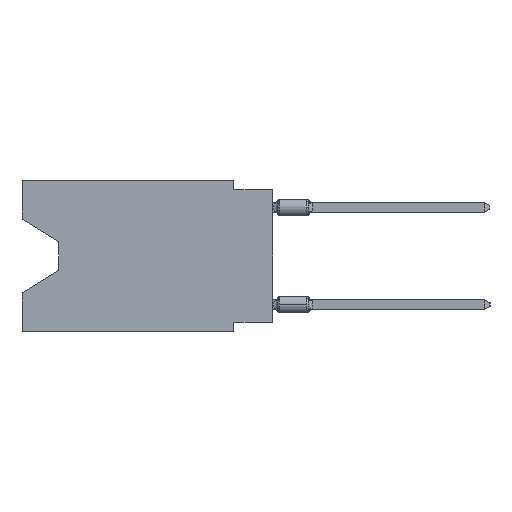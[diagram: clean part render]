
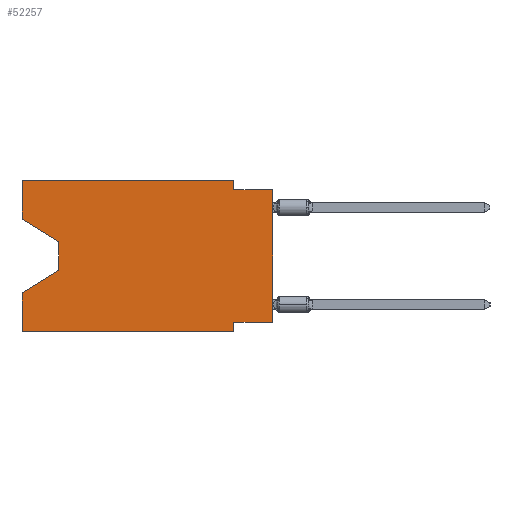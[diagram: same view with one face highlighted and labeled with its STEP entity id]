
A CAD part, left-side view. The second image highlights one B-rep face of the part: STEP entity #52257.
In plain terms, the highlighted planar face has unit normal (-1, 0, 0).
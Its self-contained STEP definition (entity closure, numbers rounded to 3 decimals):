
#366 = EDGE_CURVE ( 'NONE', #55638, #28346, #46553, .T. ) ;
#1294 = VECTOR ( 'NONE', #20960, 1000. ) ;
#1866 = VERTEX_POINT ( 'NONE', #36059 ) ;
#1870 = ORIENTED_EDGE ( 'NONE', *, *, #53201, .T. ) ;
#2819 = ORIENTED_EDGE ( 'NONE', *, *, #52890, .T. ) ;
#2922 = EDGE_CURVE ( 'NONE', #54757, #55638, #57421, .T. ) ;
#4633 = PLANE ( 'NONE',  #50530 ) ;
#4907 = DIRECTION ( 'NONE',  ( 0., -0.855, -0.519 ) ) ;
#5307 = ORIENTED_EDGE ( 'NONE', *, *, #57145, .F. ) ;
#5573 = DIRECTION ( 'NONE',  ( 0., 0., 1. ) ) ;
#8539 = EDGE_CURVE ( 'NONE', #25797, #28346, #11814, .T. ) ;
#8674 = VECTOR ( 'NONE', #58001, 1000. ) ;
#8741 = ORIENTED_EDGE ( 'NONE', *, *, #15308, .F. ) ;
#9091 = DIRECTION ( 'NONE',  ( 0., -1., 0. ) ) ;
#10360 = VECTOR ( 'NONE', #36535, 1000. ) ;
#11377 = LINE ( 'NONE', #33878, #1294 ) ;
#11814 = LINE ( 'NONE', #14172, #19852 ) ;
#13348 = LINE ( 'NONE', #13637, #20551 ) ;
#13607 = CARTESIAN_POINT ( 'NONE',  ( 0., 13.97, -5.893 ) ) ;
#13637 = CARTESIAN_POINT ( 'NONE',  ( 0., 13.97, -4.013 ) ) ;
#13999 = CARTESIAN_POINT ( 'NONE',  ( 0., 2.54, -9.271 ) ) ;
#14172 = CARTESIAN_POINT ( 'NONE',  ( 0., 16.383, -9.906 ) ) ;
#14525 = DIRECTION ( 'NONE',  ( 0., 0., -1. ) ) ;
#15308 = EDGE_CURVE ( 'NONE', #23628, #32396, #30464, .T. ) ;
#16173 = EDGE_CURVE ( 'NONE', #55126, #47197, #18011, .T. ) ;
#16391 = CARTESIAN_POINT ( 'NONE',  ( 0., 0., -9.271 ) ) ;
#16395 = CARTESIAN_POINT ( 'NONE',  ( 0., 2.54, -9.906 ) ) ;
#16447 = EDGE_CURVE ( 'NONE', #45241, #1866, #11377, .T. ) ;
#18011 = LINE ( 'NONE', #49432, #23312 ) ;
#18256 = CARTESIAN_POINT ( 'NONE',  ( 0., 2.54, -9.906 ) ) ;
#19359 = EDGE_CURVE ( 'NONE', #47197, #27373, #24805, .T. ) ;
#19852 = VECTOR ( 'NONE', #9091, 1000. ) ;
#20551 = VECTOR ( 'NONE', #14525, 1000. ) ;
#20960 = DIRECTION ( 'NONE',  ( 0., 0.855, -0.519 ) ) ;
#21456 = ORIENTED_EDGE ( 'NONE', *, *, #45015, .F. ) ;
#22072 = ORIENTED_EDGE ( 'NONE', *, *, #16447, .T. ) ;
#23112 = ORIENTED_EDGE ( 'NONE', *, *, #19359, .F. ) ;
#23312 = VECTOR ( 'NONE', #57852, 1000. ) ;
#23628 = VERTEX_POINT ( 'NONE', #31144 ) ;
#24805 = LINE ( 'NONE', #33212, #38998 ) ;
#25764 = VECTOR ( 'NONE', #4907, 1000. ) ;
#25797 = VERTEX_POINT ( 'NONE', #49208 ) ;
#27012 = VERTEX_POINT ( 'NONE', #33206 ) ;
#27245 = VECTOR ( 'NONE', #5573, 1000. ) ;
#27270 = CARTESIAN_POINT ( 'NONE',  ( 0., 16.383, -2.546 ) ) ;
#27373 = VERTEX_POINT ( 'NONE', #54974 ) ;
#28013 = VECTOR ( 'NONE', #39157, 1000. ) ;
#28346 = VERTEX_POINT ( 'NONE', #16395 ) ;
#28351 = CARTESIAN_POINT ( 'NONE',  ( 0., 16.383, 0. ) ) ;
#29977 = ORIENTED_EDGE ( 'NONE', *, *, #35208, .T. ) ;
#30464 = LINE ( 'NONE', #39748, #28013 ) ;
#31144 = CARTESIAN_POINT ( 'NONE',  ( 0., 2.54, -0.635 ) ) ;
#31283 = ORIENTED_EDGE ( 'NONE', *, *, #2922, .F. ) ;
#31454 = ORIENTED_EDGE ( 'NONE', *, *, #16173, .F. ) ;
#31615 = LINE ( 'NONE', #41485, #25764 ) ;
#32214 = DIRECTION ( 'NONE',  ( 1., 0., 0. ) ) ;
#32396 = VERTEX_POINT ( 'NONE', #38768 ) ;
#33206 = CARTESIAN_POINT ( 'NONE',  ( 0., 13.97, -4.013 ) ) ;
#33212 = CARTESIAN_POINT ( 'NONE',  ( 0., 16.383, 0. ) ) ;
#33878 = CARTESIAN_POINT ( 'NONE',  ( 0., 13.97, -5.893 ) ) ;
#34643 = CARTESIAN_POINT ( 'NONE',  ( 0., 2.54, 0. ) ) ;
#35162 = CARTESIAN_POINT ( 'NONE',  ( 0., 0., 0. ) ) ;
#35208 = EDGE_CURVE ( 'NONE', #27012, #45241, #13348, .T. ) ;
#36059 = CARTESIAN_POINT ( 'NONE',  ( 0., 16.383, -7.36 ) ) ;
#36255 = ORIENTED_EDGE ( 'NONE', *, *, #366, .F. ) ;
#36535 = DIRECTION ( 'NONE',  ( 0., 0., -1. ) ) ;
#38768 = CARTESIAN_POINT ( 'NONE',  ( 0., 0., -0.635 ) ) ;
#38841 = DIRECTION ( 'NONE',  ( 0., 0., -1. ) ) ;
#38998 = VECTOR ( 'NONE', #43061, 1000. ) ;
#39157 = DIRECTION ( 'NONE',  ( 0., -1., 0. ) ) ;
#39356 = DIRECTION ( 'NONE',  ( 0., 0., 1. ) ) ;
#39748 = CARTESIAN_POINT ( 'NONE',  ( 0., 0., -0.635 ) ) ;
#41485 = CARTESIAN_POINT ( 'NONE',  ( 0., 16.383, -2.546 ) ) ;
#42362 = VECTOR ( 'NONE', #38841, 1000. ) ;
#42382 = CARTESIAN_POINT ( 'NONE',  ( 0., 16.383, 0. ) ) ;
#43061 = DIRECTION ( 'NONE',  ( 0., -1., 0. ) ) ;
#43305 = LINE ( 'NONE', #28351, #27245 ) ;
#44353 = CARTESIAN_POINT ( 'NONE',  ( 0., 16.383, 0. ) ) ;
#45015 = EDGE_CURVE ( 'NONE', #25797, #1866, #43305, .T. ) ;
#45241 = VERTEX_POINT ( 'NONE', #13607 ) ;
#45657 = CARTESIAN_POINT ( 'NONE',  ( 0., 0., -9.271 ) ) ;
#45664 = FACE_OUTER_BOUND ( 'NONE', #56021, .T. ) ;
#46553 = LINE ( 'NONE', #18256, #10360 ) ;
#47197 = VERTEX_POINT ( 'NONE', #44353 ) ;
#49208 = CARTESIAN_POINT ( 'NONE',  ( 0., 16.383, -9.906 ) ) ;
#49432 = CARTESIAN_POINT ( 'NONE',  ( 0., 16.383, 0. ) ) ;
#50451 = DIRECTION ( 'NONE',  ( 0., 0., -1. ) ) ;
#50530 = AXIS2_PLACEMENT_3D ( 'NONE', #42382, #32214, #50451 ) ;
#52257 = ADVANCED_FACE ( 'NONE', ( #45664 ), #4633, .F. ) ;
#52329 = ORIENTED_EDGE ( 'NONE', *, *, #8539, .T. ) ;
#52890 = EDGE_CURVE ( 'NONE', #55126, #27012, #31615, .T. ) ;
#53201 = EDGE_CURVE ( 'NONE', #54757, #32396, #57893, .T. ) ;
#53494 = VECTOR ( 'NONE', #39356, 1000. ) ;
#54757 = VERTEX_POINT ( 'NONE', #45657 ) ;
#54974 = CARTESIAN_POINT ( 'NONE',  ( 0., 2.54, 0. ) ) ;
#55126 = VERTEX_POINT ( 'NONE', #27270 ) ;
#55638 = VERTEX_POINT ( 'NONE', #13999 ) ;
#56021 = EDGE_LOOP ( 'NONE', ( #2819, #29977, #22072, #21456, #52329, #36255, #31283, #1870, #8741, #5307, #23112, #31454 ) ) ;
#56497 = LINE ( 'NONE', #34643, #42362 ) ;
#57145 = EDGE_CURVE ( 'NONE', #27373, #23628, #56497, .T. ) ;
#57421 = LINE ( 'NONE', #16391, #8674 ) ;
#57852 = DIRECTION ( 'NONE',  ( 0., 0., 1. ) ) ;
#57893 = LINE ( 'NONE', #35162, #53494 ) ;
#58001 = DIRECTION ( 'NONE',  ( 0., 1., 0. ) ) ;
